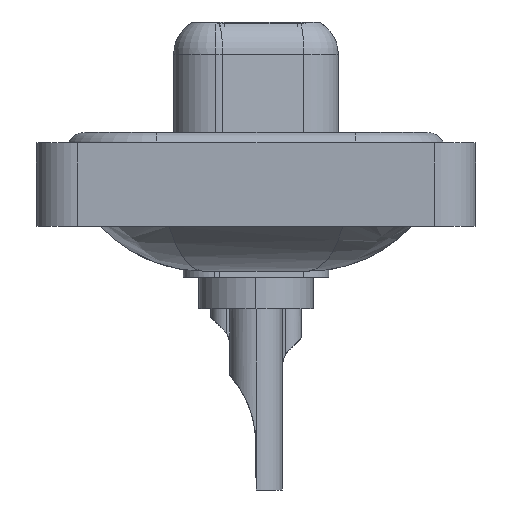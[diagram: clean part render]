
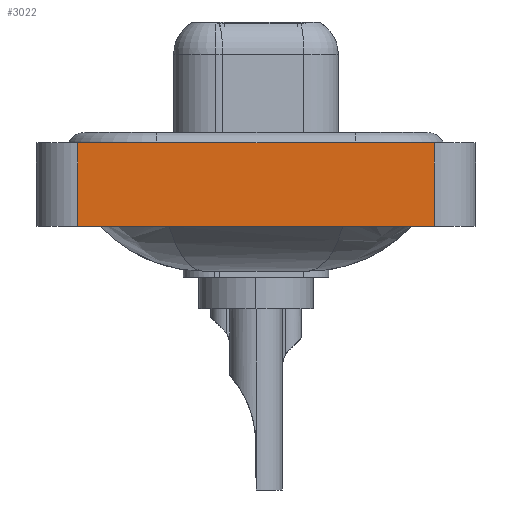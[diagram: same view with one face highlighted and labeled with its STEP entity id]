
A CAD part, left-side view. The second image highlights one B-rep face of the part: STEP entity #3022.
In plain terms, the highlighted planar face has unit normal (-1, 0, 0).
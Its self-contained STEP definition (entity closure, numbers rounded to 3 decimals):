
#293 = AXIS2_PLACEMENT_3D ( 'NONE', #9699, #16166, #3181 ) ;
#593 = ORIENTED_EDGE ( 'NONE', *, *, #20700, .F. ) ;
#943 = DIRECTION ( 'NONE',  ( 0., -1., 0. ) ) ;
#1604 = EDGE_CURVE ( 'NONE', #8332, #3968, #8470, .T. ) ;
#1967 = CARTESIAN_POINT ( 'NONE',  ( -7.35, -8.55, 0.4 ) ) ;
#3008 = DIRECTION ( 'NONE',  ( 0., 0., 1. ) ) ;
#3022 = ADVANCED_FACE ( 'NONE', ( #17756 ), #17958, .T. ) ;
#3181 = DIRECTION ( 'NONE',  ( 0., 0., 1. ) ) ;
#3428 = LINE ( 'NONE', #19594, #12809 ) ;
#3780 = DIRECTION ( 'NONE',  ( 0., 0., 1. ) ) ;
#3925 = ORIENTED_EDGE ( 'NONE', *, *, #1604, .T. ) ;
#3968 = VERTEX_POINT ( 'NONE', #1967 ) ;
#4038 = VECTOR ( 'NONE', #943, 1000. ) ;
#4999 = ORIENTED_EDGE ( 'NONE', *, *, #14773, .F. ) ;
#7492 = VECTOR ( 'NONE', #12432, 1000. ) ;
#8074 = CARTESIAN_POINT ( 'NONE',  ( -7.35, -8.55, -3.6 ) ) ;
#8120 = CARTESIAN_POINT ( 'NONE',  ( -7.35, 8.55, -3.6 ) ) ;
#8332 = VERTEX_POINT ( 'NONE', #8074 ) ;
#8470 = LINE ( 'NONE', #19946, #12277 ) ;
#9139 = CARTESIAN_POINT ( 'NONE',  ( -7.35, -8.55, 0.4 ) ) ;
#9699 = CARTESIAN_POINT ( 'NONE',  ( -7.35, -8.55, -3.6 ) ) ;
#11225 = EDGE_LOOP ( 'NONE', ( #3925, #593, #4999, #11538 ) ) ;
#11538 = ORIENTED_EDGE ( 'NONE', *, *, #11975, .T. ) ;
#11975 = EDGE_CURVE ( 'NONE', #13976, #8332, #14016, .T. ) ;
#12277 = VECTOR ( 'NONE', #3780, 1000. ) ;
#12432 = DIRECTION ( 'NONE',  ( 0., -1., 0. ) ) ;
#12809 = VECTOR ( 'NONE', #3008, 1000. ) ;
#13976 = VERTEX_POINT ( 'NONE', #8120 ) ;
#14016 = LINE ( 'NONE', #19297, #7492 ) ;
#14035 = LINE ( 'NONE', #9139, #4038 ) ;
#14773 = EDGE_CURVE ( 'NONE', #13976, #17741, #3428, .T. ) ;
#16166 = DIRECTION ( 'NONE',  ( -1., 0., 0. ) ) ;
#17741 = VERTEX_POINT ( 'NONE', #18243 ) ;
#17756 = FACE_OUTER_BOUND ( 'NONE', #11225, .T. ) ;
#17958 = PLANE ( 'NONE',  #293 ) ;
#18243 = CARTESIAN_POINT ( 'NONE',  ( -7.35, 8.55, 0.4 ) ) ;
#19297 = CARTESIAN_POINT ( 'NONE',  ( -7.35, -8.55, -3.6 ) ) ;
#19594 = CARTESIAN_POINT ( 'NONE',  ( -7.35, 8.55, -3.6 ) ) ;
#19946 = CARTESIAN_POINT ( 'NONE',  ( -7.35, -8.55, -3.6 ) ) ;
#20700 = EDGE_CURVE ( 'NONE', #17741, #3968, #14035, .T. ) ;
